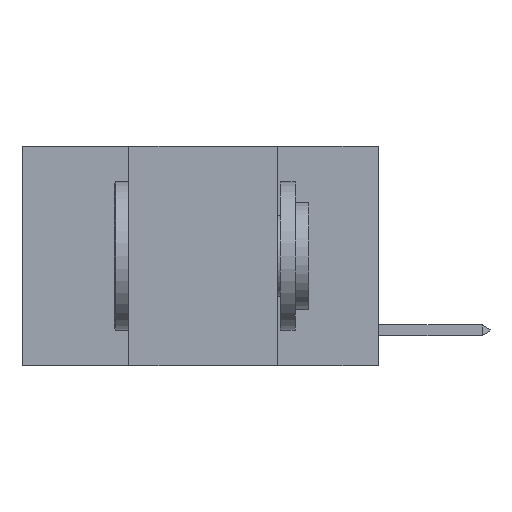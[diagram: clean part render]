
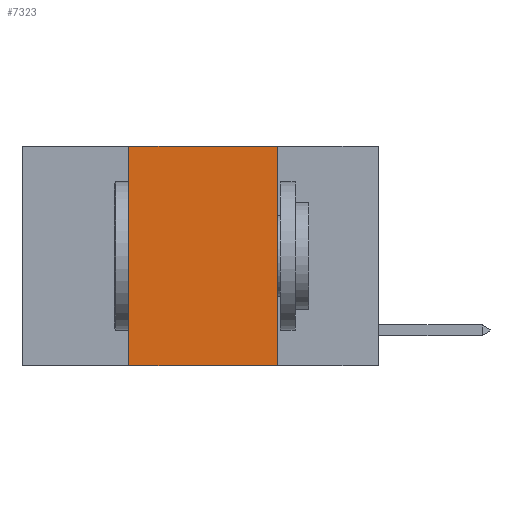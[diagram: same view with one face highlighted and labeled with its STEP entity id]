
A CAD part, left-side view. The second image highlights one B-rep face of the part: STEP entity #7323.
In plain terms, the highlighted planar face has unit normal (-1, 0, 0).
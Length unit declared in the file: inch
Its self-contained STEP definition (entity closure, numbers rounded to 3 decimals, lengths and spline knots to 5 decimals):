
#368 = DIRECTION ( 'NONE',  ( 0., 0., -1. ) ) ;
#470 = VERTEX_POINT ( 'NONE', #9746 ) ;
#693 = CARTESIAN_POINT ( 'NONE',  ( 0., 0.6, -0.37 ) ) ;
#758 = LINE ( 'NONE', #693, #8019 ) ;
#983 = EDGE_CURVE ( 'NONE', #13542, #8838, #758, .T. ) ;
#1011 = VECTOR ( 'NONE', #12007, 39.37008 ) ;
#1431 = EDGE_CURVE ( 'NONE', #3867, #470, #11352, .T. ) ;
#1822 = EDGE_LOOP ( 'NONE', ( #11220, #5416, #12551, #11507 ) ) ;
#2042 = CARTESIAN_POINT ( 'NONE',  ( 0., 0.17, -0.37 ) ) ;
#3515 = CARTESIAN_POINT ( 'NONE',  ( 0., 0.17, 0. ) ) ;
#3599 = CARTESIAN_POINT ( 'NONE',  ( 0., 0.42, 0. ) ) ;
#3771 = CARTESIAN_POINT ( 'NONE',  ( 0., 0.6, 0. ) ) ;
#3867 = VERTEX_POINT ( 'NONE', #3599 ) ;
#4050 = DIRECTION ( 'NONE',  ( 0., -1., 0. ) ) ;
#4335 = EDGE_CURVE ( 'NONE', #470, #8838, #6674, .T. ) ;
#4516 = CARTESIAN_POINT ( 'NONE',  ( 0., 0.6, 0. ) ) ;
#5310 = VECTOR ( 'NONE', #4050, 39.37008 ) ;
#5416 = ORIENTED_EDGE ( 'NONE', *, *, #1431, .F. ) ;
#6397 = AXIS2_PLACEMENT_3D ( 'NONE', #4516, #7852, #368 ) ;
#6674 = LINE ( 'NONE', #3515, #1011 ) ;
#6989 = DIRECTION ( 'NONE',  ( 0., -1., 0. ) ) ;
#7323 = ADVANCED_FACE ( 'NONE', ( #11137 ), #10158, .F. ) ;
#7450 = DIRECTION ( 'NONE',  ( 0., 0., 1. ) ) ;
#7527 = CARTESIAN_POINT ( 'NONE',  ( 0., 0.42, 0. ) ) ;
#7852 = DIRECTION ( 'NONE',  ( 1., 0., 0. ) ) ;
#8019 = VECTOR ( 'NONE', #6989, 39.37008 ) ;
#8042 = VECTOR ( 'NONE', #7450, 39.37008 ) ;
#8838 = VERTEX_POINT ( 'NONE', #2042 ) ;
#9746 = CARTESIAN_POINT ( 'NONE',  ( 0., 0.17, 0. ) ) ;
#9927 = EDGE_CURVE ( 'NONE', #13542, #3867, #12991, .T. ) ;
#10158 = PLANE ( 'NONE',  #6397 ) ;
#11137 = FACE_OUTER_BOUND ( 'NONE', #1822, .T. ) ;
#11220 = ORIENTED_EDGE ( 'NONE', *, *, #4335, .F. ) ;
#11352 = LINE ( 'NONE', #3771, #5310 ) ;
#11507 = ORIENTED_EDGE ( 'NONE', *, *, #983, .T. ) ;
#12007 = DIRECTION ( 'NONE',  ( 0., 0., -1. ) ) ;
#12551 = ORIENTED_EDGE ( 'NONE', *, *, #9927, .F. ) ;
#12991 = LINE ( 'NONE', #7527, #8042 ) ;
#13542 = VERTEX_POINT ( 'NONE', #13685 ) ;
#13685 = CARTESIAN_POINT ( 'NONE',  ( 0., 0.42, -0.37 ) ) ;
